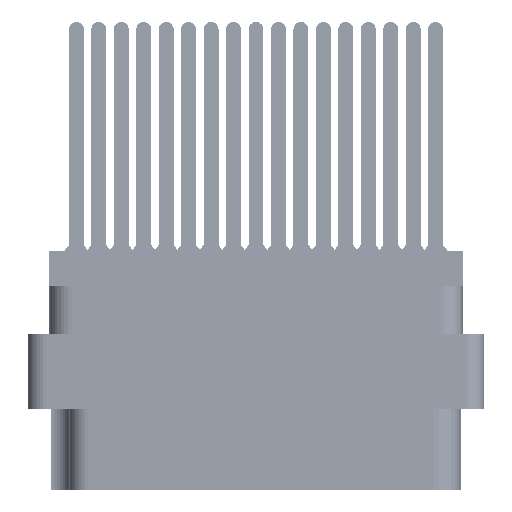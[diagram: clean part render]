
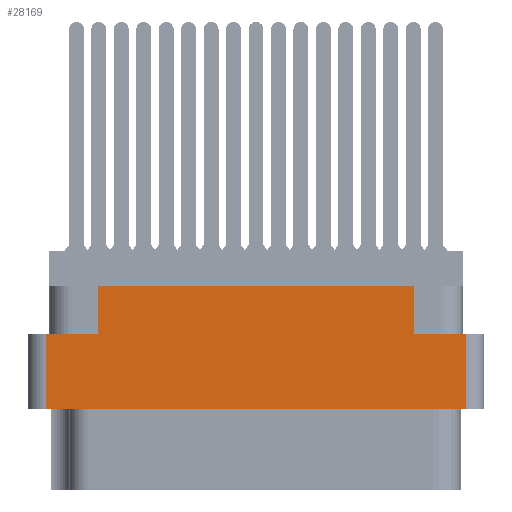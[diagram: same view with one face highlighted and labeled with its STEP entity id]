
A CAD part, left-side view. The second image highlights one B-rep face of the part: STEP entity #28169.
In plain terms, the highlighted planar face has unit normal (-1, 0, 0).
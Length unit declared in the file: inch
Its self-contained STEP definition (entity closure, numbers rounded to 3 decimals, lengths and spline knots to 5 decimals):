
#1535 = DIRECTION ( 'NONE',  ( 0., 1., 0. ) ) ;
#1925 = VERTEX_POINT ( 'NONE', #68081 ) ;
#2261 = CARTESIAN_POINT ( 'NONE',  ( -1.375, 0.7625, -0.117 ) ) ;
#3680 = LINE ( 'NONE', #47333, #26742 ) ;
#5323 = CARTESIAN_POINT ( 'NONE',  ( -1.375, -0.7625, -0.798 ) ) ;
#8211 = VERTEX_POINT ( 'NONE', #13588 ) ;
#9176 = DIRECTION ( 'NONE',  ( 0., -1., 0. ) ) ;
#10392 = CARTESIAN_POINT ( 'NONE',  ( -1.375, 0., -0.277 ) ) ;
#11320 = EDGE_CURVE ( 'NONE', #1925, #50239, #43281, .T. ) ;
#13588 = CARTESIAN_POINT ( 'NONE',  ( -1.375, -0.5285, -0.117 ) ) ;
#16863 = CARTESIAN_POINT ( 'NONE',  ( -1.375, -0.7005, -0.529 ) ) ;
#16939 = VECTOR ( 'NONE', #1535, 39.37008 ) ;
#19450 = DIRECTION ( 'NONE',  ( 0., 0., 1. ) ) ;
#20361 = DIRECTION ( 'NONE',  ( -1., 0., 0. ) ) ;
#21995 = LINE ( 'NONE', #74562, #36196 ) ;
#25583 = VERTEX_POINT ( 'NONE', #16863 ) ;
#26742 = VECTOR ( 'NONE', #83617, 39.37008 ) ;
#28169 = ADVANCED_FACE ( 'NONE', ( #68581 ), #89079, .T. ) ;
#30055 = LINE ( 'NONE', #36323, #42126 ) ;
#30884 = VERTEX_POINT ( 'NONE', #37216 ) ;
#31634 = EDGE_CURVE ( 'NONE', #69546, #55913, #44921, .T. ) ;
#33874 = EDGE_CURVE ( 'NONE', #30884, #69546, #60931, .T. ) ;
#34921 = ORIENTED_EDGE ( 'NONE', *, *, #31634, .F. ) ;
#35887 = CARTESIAN_POINT ( 'NONE',  ( -1.375, 0., -0.529 ) ) ;
#36087 = VECTOR ( 'NONE', #71965, 39.37008 ) ;
#36196 = VECTOR ( 'NONE', #59906, 39.37008 ) ;
#36323 = CARTESIAN_POINT ( 'NONE',  ( -1.375, -0.5285, -0.277 ) ) ;
#37216 = CARTESIAN_POINT ( 'NONE',  ( -1.375, 0.7005, -0.277 ) ) ;
#37580 = DIRECTION ( 'NONE',  ( 0., -1., 0. ) ) ;
#38540 = ORIENTED_EDGE ( 'NONE', *, *, #54620, .F. ) ;
#39437 = ORIENTED_EDGE ( 'NONE', *, *, #55138, .F. ) ;
#42126 = VECTOR ( 'NONE', #78818, 39.37008 ) ;
#43281 = LINE ( 'NONE', #57795, #88021 ) ;
#43963 = DIRECTION ( 'NONE',  ( 0., -1., 0. ) ) ;
#44921 = LINE ( 'NONE', #50903, #36087 ) ;
#46525 = ORIENTED_EDGE ( 'NONE', *, *, #11320, .F. ) ;
#46563 = VECTOR ( 'NONE', #43963, 39.37008 ) ;
#47333 = CARTESIAN_POINT ( 'NONE',  ( -1.375, -0.7005, -0.798 ) ) ;
#50239 = VERTEX_POINT ( 'NONE', #79198 ) ;
#50303 = EDGE_CURVE ( 'NONE', #30884, #81391, #21995, .T. ) ;
#50843 = ORIENTED_EDGE ( 'NONE', *, *, #50303, .T. ) ;
#50903 = CARTESIAN_POINT ( 'NONE',  ( -1.375, 0.5285, -0.277 ) ) ;
#52568 = CARTESIAN_POINT ( 'NONE',  ( -1.375, 0.5285, -0.117 ) ) ;
#54620 = EDGE_CURVE ( 'NONE', #55913, #8211, #60722, .T. ) ;
#55138 = EDGE_CURVE ( 'NONE', #25583, #81391, #61804, .T. ) ;
#55913 = VERTEX_POINT ( 'NONE', #52568 ) ;
#57575 = ORIENTED_EDGE ( 'NONE', *, *, #58776, .T. ) ;
#57795 = CARTESIAN_POINT ( 'NONE',  ( -1.375, 0., -0.277 ) ) ;
#58776 = EDGE_CURVE ( 'NONE', #25583, #50239, #3680, .T. ) ;
#59906 = DIRECTION ( 'NONE',  ( 0., 0., -1. ) ) ;
#60722 = LINE ( 'NONE', #2261, #46563 ) ;
#60931 = LINE ( 'NONE', #10392, #67543 ) ;
#61804 = LINE ( 'NONE', #35887, #16939 ) ;
#62820 = CARTESIAN_POINT ( 'NONE',  ( -1.375, 0.7005, -0.529 ) ) ;
#65499 = EDGE_CURVE ( 'NONE', #1925, #8211, #30055, .T. ) ;
#67425 = ORIENTED_EDGE ( 'NONE', *, *, #65499, .T. ) ;
#67543 = VECTOR ( 'NONE', #9176, 39.37008 ) ;
#68081 = CARTESIAN_POINT ( 'NONE',  ( -1.375, -0.5285, -0.277 ) ) ;
#68581 = FACE_OUTER_BOUND ( 'NONE', #70308, .T. ) ;
#69546 = VERTEX_POINT ( 'NONE', #77049 ) ;
#70308 = EDGE_LOOP ( 'NONE', ( #79625, #50843, #39437, #57575, #46525, #67425, #38540, #34921 ) ) ;
#71965 = DIRECTION ( 'NONE',  ( 0., 0., 1. ) ) ;
#74562 = CARTESIAN_POINT ( 'NONE',  ( -1.375, 0.7005, -0.798 ) ) ;
#77049 = CARTESIAN_POINT ( 'NONE',  ( -1.375, 0.5285, -0.277 ) ) ;
#78818 = DIRECTION ( 'NONE',  ( 0., 0., 1. ) ) ;
#79198 = CARTESIAN_POINT ( 'NONE',  ( -1.375, -0.7005, -0.277 ) ) ;
#79625 = ORIENTED_EDGE ( 'NONE', *, *, #33874, .F. ) ;
#81391 = VERTEX_POINT ( 'NONE', #62820 ) ;
#83617 = DIRECTION ( 'NONE',  ( 0., 0., 1. ) ) ;
#84514 = AXIS2_PLACEMENT_3D ( 'NONE', #5323, #20361, #19450 ) ;
#88021 = VECTOR ( 'NONE', #37580, 39.37008 ) ;
#89079 = PLANE ( 'NONE',  #84514 ) ;
